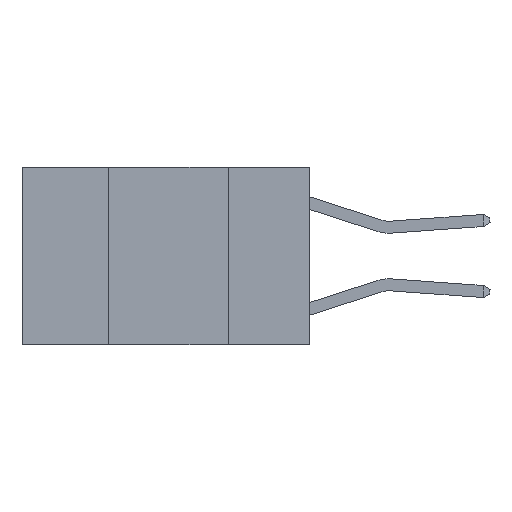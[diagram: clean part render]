
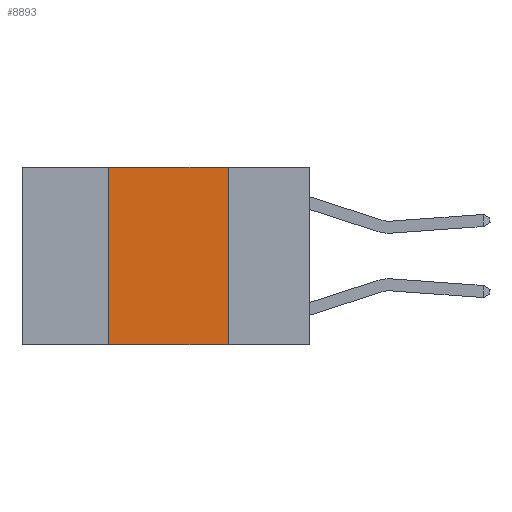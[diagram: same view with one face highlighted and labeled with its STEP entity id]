
A CAD part, left-side view. The second image highlights one B-rep face of the part: STEP entity #8893.
In plain terms, the highlighted planar face has unit normal (-1, 0, 0).
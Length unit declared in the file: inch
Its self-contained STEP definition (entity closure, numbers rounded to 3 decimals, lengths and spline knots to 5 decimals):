
#142 = FACE_OUTER_BOUND ( 'NONE', #6210, .T. ) ;
#934 = AXIS2_PLACEMENT_3D ( 'NONE', #8754, #1138, #6984 ) ;
#967 = PLANE ( 'NONE',  #934 ) ;
#1062 = ORIENTED_EDGE ( 'NONE', *, *, #1659, .F. ) ;
#1098 = VERTEX_POINT ( 'NONE', #2216 ) ;
#1138 = DIRECTION ( 'NONE',  ( 1., 0., 0. ) ) ;
#1283 = DIRECTION ( 'NONE',  ( 0., 0., -1. ) ) ;
#1473 = VERTEX_POINT ( 'NONE', #8467 ) ;
#1659 = EDGE_CURVE ( 'NONE', #5321, #1473, #7210, .T. ) ;
#2216 = CARTESIAN_POINT ( 'NONE',  ( 0., 0.17, 0. ) ) ;
#2508 = DIRECTION ( 'NONE',  ( 0., -1., 0. ) ) ;
#2713 = VECTOR ( 'NONE', #1283, 39.37008 ) ;
#3449 = CARTESIAN_POINT ( 'NONE',  ( 0., 0.17, -0.37 ) ) ;
#4018 = EDGE_CURVE ( 'NONE', #1473, #1098, #5676, .T. ) ;
#5182 = ORIENTED_EDGE ( 'NONE', *, *, #9145, .T. ) ;
#5321 = VERTEX_POINT ( 'NONE', #10105 ) ;
#5459 = DIRECTION ( 'NONE',  ( 0., -1., 0. ) ) ;
#5676 = LINE ( 'NONE', #9112, #9227 ) ;
#5715 = VECTOR ( 'NONE', #8117, 39.37008 ) ;
#6210 = EDGE_LOOP ( 'NONE', ( #7607, #9443, #1062, #5182 ) ) ;
#6753 = LINE ( 'NONE', #11073, #10810 ) ;
#6984 = DIRECTION ( 'NONE',  ( 0., 0., -1. ) ) ;
#7210 = LINE ( 'NONE', #10469, #5715 ) ;
#7607 = ORIENTED_EDGE ( 'NONE', *, *, #8332, .F. ) ;
#8093 = CARTESIAN_POINT ( 'NONE',  ( 0., 0.17, 0. ) ) ;
#8117 = DIRECTION ( 'NONE',  ( 0., 0., 1. ) ) ;
#8332 = EDGE_CURVE ( 'NONE', #1098, #9759, #9015, .T. ) ;
#8467 = CARTESIAN_POINT ( 'NONE',  ( 0., 0.42, 0. ) ) ;
#8754 = CARTESIAN_POINT ( 'NONE',  ( 0., 0.6, 0. ) ) ;
#8893 = ADVANCED_FACE ( 'NONE', ( #142 ), #967, .F. ) ;
#9015 = LINE ( 'NONE', #8093, #2713 ) ;
#9112 = CARTESIAN_POINT ( 'NONE',  ( 0., 0.6, 0. ) ) ;
#9145 = EDGE_CURVE ( 'NONE', #5321, #9759, #6753, .T. ) ;
#9227 = VECTOR ( 'NONE', #5459, 39.37008 ) ;
#9443 = ORIENTED_EDGE ( 'NONE', *, *, #4018, .F. ) ;
#9759 = VERTEX_POINT ( 'NONE', #3449 ) ;
#10105 = CARTESIAN_POINT ( 'NONE',  ( 0., 0.42, -0.37 ) ) ;
#10469 = CARTESIAN_POINT ( 'NONE',  ( 0., 0.42, 0. ) ) ;
#10810 = VECTOR ( 'NONE', #2508, 39.37008 ) ;
#11073 = CARTESIAN_POINT ( 'NONE',  ( 0., 0.6, -0.37 ) ) ;
